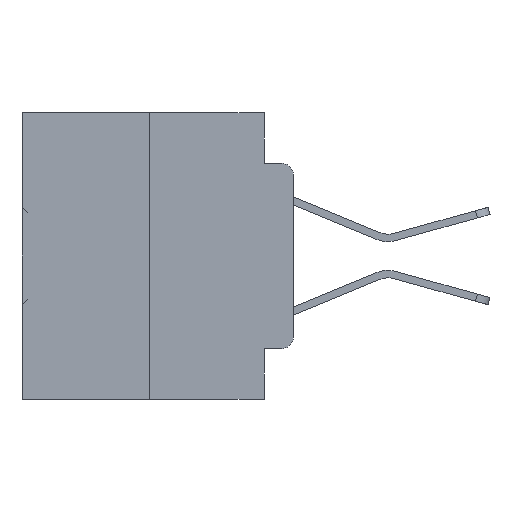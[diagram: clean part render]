
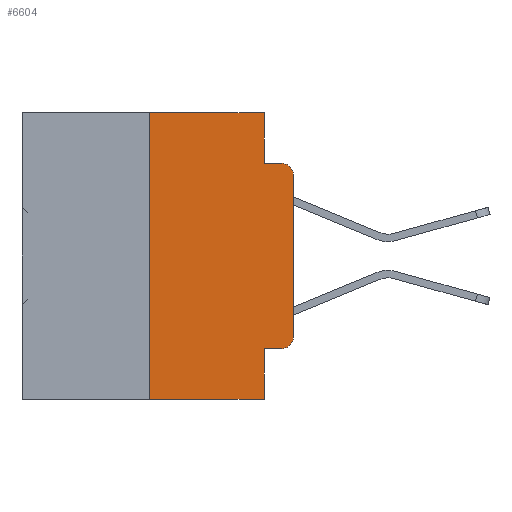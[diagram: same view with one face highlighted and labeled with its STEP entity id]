
A CAD part, left-side view. The second image highlights one B-rep face of the part: STEP entity #6604.
In plain terms, the highlighted planar face has unit normal (-1, 0, 0).
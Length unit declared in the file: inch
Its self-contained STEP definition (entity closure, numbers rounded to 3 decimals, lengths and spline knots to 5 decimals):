
#822 = EDGE_CURVE ( 'NONE', #27983, #12421, #29968, .T. ) ;
#843 = DIRECTION ( 'NONE',  ( 0., 0., -1. ) ) ;
#1243 = DIRECTION ( 'NONE',  ( 0., 0., -1. ) ) ;
#2326 = DIRECTION ( 'NONE',  ( 0., 0., -1. ) ) ;
#2445 = LINE ( 'NONE', #28754, #8541 ) ;
#2629 = CARTESIAN_POINT ( 'NONE',  ( 0., 0., 0. ) ) ;
#3231 = CARTESIAN_POINT ( 'NONE',  ( 0., 0.02, -0.0885 ) ) ;
#3891 = CARTESIAN_POINT ( 'NONE',  ( 0., 0.051, 0. ) ) ;
#3981 = VECTOR ( 'NONE', #4065, 39.37008 ) ;
#4065 = DIRECTION ( 'NONE',  ( 0., -1., 0. ) ) ;
#4439 = CARTESIAN_POINT ( 'NONE',  ( 0., 0.02, -0.3915 ) ) ;
#5654 = EDGE_CURVE ( 'NONE', #15600, #33812, #11516, .T. ) ;
#6604 = ADVANCED_FACE ( 'NONE', ( #30816 ), #23244, .F. ) ;
#7608 = VERTEX_POINT ( 'NONE', #24424 ) ;
#8484 = VERTEX_POINT ( 'NONE', #27485 ) ;
#8541 = VECTOR ( 'NONE', #31563, 39.37008 ) ;
#8810 = CARTESIAN_POINT ( 'NONE',  ( 0., 0.051, -0.4115 ) ) ;
#8891 = ORIENTED_EDGE ( 'NONE', *, *, #822, .T. ) ;
#8944 = LINE ( 'NONE', #31875, #3981 ) ;
#9010 = ORIENTED_EDGE ( 'NONE', *, *, #10305, .F. ) ;
#9405 = ORIENTED_EDGE ( 'NONE', *, *, #5654, .T. ) ;
#9693 = DIRECTION ( 'NONE',  ( 0., -1., 0. ) ) ;
#9801 = ORIENTED_EDGE ( 'NONE', *, *, #28283, .F. ) ;
#10102 = CARTESIAN_POINT ( 'NONE',  ( 0., 0.051, 0. ) ) ;
#10199 = CARTESIAN_POINT ( 'NONE',  ( 0., 0.25, 0. ) ) ;
#10305 = EDGE_CURVE ( 'NONE', #7608, #8484, #2445, .T. ) ;
#10428 = VERTEX_POINT ( 'NONE', #8810 ) ;
#10665 = EDGE_CURVE ( 'NONE', #10428, #12421, #19160, .T. ) ;
#11379 = VECTOR ( 'NONE', #13542, 39.37008 ) ;
#11516 = CIRCLE ( 'NONE', #31895, 0.02 ) ;
#12029 = AXIS2_PLACEMENT_3D ( 'NONE', #34132, #19854, #843 ) ;
#12350 = DIRECTION ( 'NONE',  ( -1., 0., 0. ) ) ;
#12421 = VERTEX_POINT ( 'NONE', #24558 ) ;
#12512 = DIRECTION ( 'NONE',  ( 0., -1., 0. ) ) ;
#12535 = DIRECTION ( 'NONE',  ( 0., 0., -1. ) ) ;
#13139 = CARTESIAN_POINT ( 'NONE',  ( 0., 0.25, -0.5 ) ) ;
#13542 = DIRECTION ( 'NONE',  ( 0., 0., 1. ) ) ;
#13611 = DIRECTION ( 'NONE',  ( -1., 0., 0. ) ) ;
#14149 = CARTESIAN_POINT ( 'NONE',  ( 0., 0.051, -0.0885 ) ) ;
#14216 = CARTESIAN_POINT ( 'NONE',  ( 0., 0., -0.1085 ) ) ;
#14353 = CARTESIAN_POINT ( 'NONE',  ( 0., 0.02, -0.1085 ) ) ;
#14856 = ORIENTED_EDGE ( 'NONE', *, *, #26547, .F. ) ;
#15600 = VERTEX_POINT ( 'NONE', #14216 ) ;
#18689 = DIRECTION ( 'NONE',  ( 0., 0., 1. ) ) ;
#18863 = EDGE_CURVE ( 'NONE', #10428, #35440, #31888, .T. ) ;
#18920 = EDGE_CURVE ( 'NONE', #35440, #34881, #31299, .T. ) ;
#18936 = EDGE_CURVE ( 'NONE', #8484, #33794, #29623, .T. ) ;
#19160 = LINE ( 'NONE', #10102, #20585 ) ;
#19479 = ORIENTED_EDGE ( 'NONE', *, *, #18936, .F. ) ;
#19854 = DIRECTION ( 'NONE',  ( 1., 0., 0. ) ) ;
#20585 = VECTOR ( 'NONE', #30590, 39.37008 ) ;
#20734 = ORIENTED_EDGE ( 'NONE', *, *, #18863, .T. ) ;
#22096 = VECTOR ( 'NONE', #18689, 39.37008 ) ;
#22304 = VECTOR ( 'NONE', #9693, 39.37008 ) ;
#22536 = EDGE_LOOP ( 'NONE', ( #36272, #9405, #14856, #19479, #9010, #9801, #8891, #25230, #20734, #30074 ) ) ;
#23244 = PLANE ( 'NONE',  #12029 ) ;
#24424 = CARTESIAN_POINT ( 'NONE',  ( 0., 0.25, 0. ) ) ;
#24558 = CARTESIAN_POINT ( 'NONE',  ( 0., 0.051, -0.5 ) ) ;
#25230 = ORIENTED_EDGE ( 'NONE', *, *, #10665, .F. ) ;
#25557 = LINE ( 'NONE', #2629, #11379 ) ;
#26477 = VECTOR ( 'NONE', #1243, 39.37008 ) ;
#26547 = EDGE_CURVE ( 'NONE', #33794, #33812, #8944, .T. ) ;
#26962 = CARTESIAN_POINT ( 'NONE',  ( 0., 0.473, -0.5 ) ) ;
#27127 = LINE ( 'NONE', #10199, #22096 ) ;
#27485 = CARTESIAN_POINT ( 'NONE',  ( 0., 0.051, 0. ) ) ;
#27983 = VERTEX_POINT ( 'NONE', #13139 ) ;
#28070 = CARTESIAN_POINT ( 'NONE',  ( 0., 0., -0.3915 ) ) ;
#28283 = EDGE_CURVE ( 'NONE', #27983, #7608, #27127, .T. ) ;
#28754 = CARTESIAN_POINT ( 'NONE',  ( 0., 0.473, 0. ) ) ;
#29623 = LINE ( 'NONE', #3891, #26477 ) ;
#29968 = LINE ( 'NONE', #26962, #33153 ) ;
#30074 = ORIENTED_EDGE ( 'NONE', *, *, #18920, .T. ) ;
#30080 = AXIS2_PLACEMENT_3D ( 'NONE', #4439, #12350, #12535 ) ;
#30083 = CARTESIAN_POINT ( 'NONE',  ( 0., 0.02, -0.4115 ) ) ;
#30177 = CARTESIAN_POINT ( 'NONE',  ( 0., 0.051, -0.4115 ) ) ;
#30481 = EDGE_CURVE ( 'NONE', #34881, #15600, #25557, .T. ) ;
#30590 = DIRECTION ( 'NONE',  ( 0., 0., -1. ) ) ;
#30816 = FACE_OUTER_BOUND ( 'NONE', #22536, .T. ) ;
#31299 = CIRCLE ( 'NONE', #30080, 0.02 ) ;
#31563 = DIRECTION ( 'NONE',  ( 0., -1., 0. ) ) ;
#31875 = CARTESIAN_POINT ( 'NONE',  ( 0., 0.051, -0.0885 ) ) ;
#31888 = LINE ( 'NONE', #30177, #22304 ) ;
#31895 = AXIS2_PLACEMENT_3D ( 'NONE', #14353, #13611, #2326 ) ;
#33153 = VECTOR ( 'NONE', #12512, 39.37008 ) ;
#33794 = VERTEX_POINT ( 'NONE', #14149 ) ;
#33812 = VERTEX_POINT ( 'NONE', #3231 ) ;
#34132 = CARTESIAN_POINT ( 'NONE',  ( 0., 0.473, 0. ) ) ;
#34881 = VERTEX_POINT ( 'NONE', #28070 ) ;
#35440 = VERTEX_POINT ( 'NONE', #30083 ) ;
#36272 = ORIENTED_EDGE ( 'NONE', *, *, #30481, .T. ) ;
